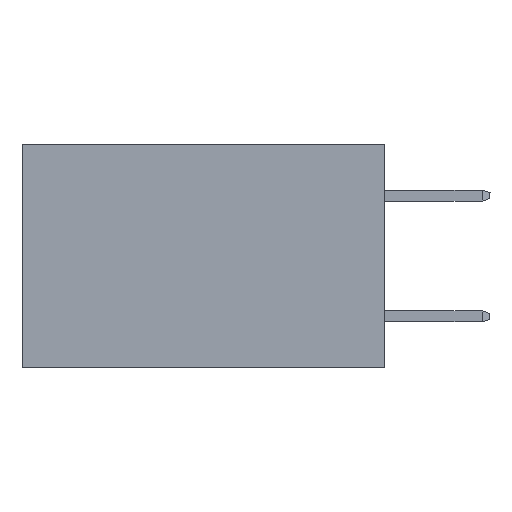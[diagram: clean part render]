
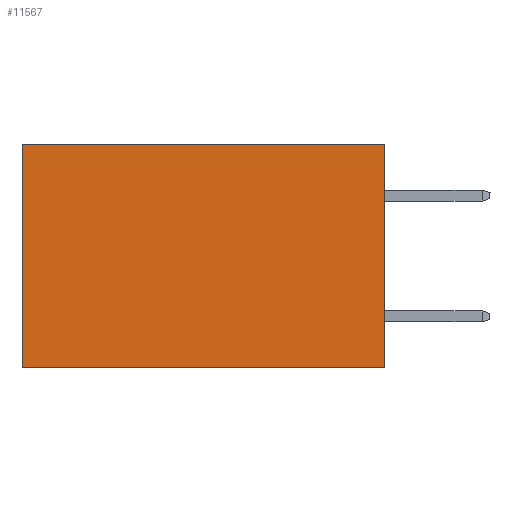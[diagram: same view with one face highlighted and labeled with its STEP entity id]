
A CAD part, left-side view. The second image highlights one B-rep face of the part: STEP entity #11567.
In plain terms, the highlighted planar face has unit normal (-1, 0, 0).
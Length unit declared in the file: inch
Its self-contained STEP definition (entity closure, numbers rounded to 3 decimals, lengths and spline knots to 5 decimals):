
#1437 = VERTEX_POINT ( 'NONE', #6724 ) ;
#1518 = VECTOR ( 'NONE', #14528, 39.37008 ) ;
#2049 = DIRECTION ( 'NONE',  ( 0., 0., -1. ) ) ;
#3207 = VECTOR ( 'NONE', #14059, 39.37008 ) ;
#3283 = VECTOR ( 'NONE', #7486, 39.37008 ) ;
#4358 = CARTESIAN_POINT ( 'NONE',  ( 0.298, 0.6, 0. ) ) ;
#4400 = EDGE_CURVE ( 'NONE', #15596, #13441, #5658, .T. ) ;
#4455 = AXIS2_PLACEMENT_3D ( 'NONE', #16062, #10477, #2049 ) ;
#5658 = LINE ( 'NONE', #14724, #1518 ) ;
#5954 = LINE ( 'NONE', #13129, #13966 ) ;
#5987 = VERTEX_POINT ( 'NONE', #13545 ) ;
#6137 = ORIENTED_EDGE ( 'NONE', *, *, #4400, .T. ) ;
#6401 = EDGE_CURVE ( 'NONE', #5987, #1437, #10658, .T. ) ;
#6724 = CARTESIAN_POINT ( 'NONE',  ( 0.298, 0., -0.37 ) ) ;
#7486 = DIRECTION ( 'NONE',  ( 0., 1., 0. ) ) ;
#7903 = EDGE_CURVE ( 'NONE', #5987, #15596, #5954, .T. ) ;
#8319 = ORIENTED_EDGE ( 'NONE', *, *, #14448, .F. ) ;
#9016 = PLANE ( 'NONE',  #4455 ) ;
#10477 = DIRECTION ( 'NONE',  ( 1., 0., 0. ) ) ;
#10658 = LINE ( 'NONE', #16275, #3207 ) ;
#10907 = ORIENTED_EDGE ( 'NONE', *, *, #6401, .F. ) ;
#11567 = ADVANCED_FACE ( 'NONE', ( #17803 ), #9016, .F. ) ;
#13129 = CARTESIAN_POINT ( 'NONE',  ( 0.298, 0., 0. ) ) ;
#13441 = VERTEX_POINT ( 'NONE', #15647 ) ;
#13545 = CARTESIAN_POINT ( 'NONE',  ( 0.298, 0., 0. ) ) ;
#13761 = DIRECTION ( 'NONE',  ( 0., 1., 0. ) ) ;
#13779 = ORIENTED_EDGE ( 'NONE', *, *, #7903, .T. ) ;
#13966 = VECTOR ( 'NONE', #13761, 39.37008 ) ;
#14059 = DIRECTION ( 'NONE',  ( 0., 0., -1. ) ) ;
#14448 = EDGE_CURVE ( 'NONE', #1437, #13441, #18161, .T. ) ;
#14528 = DIRECTION ( 'NONE',  ( 0., 0., -1. ) ) ;
#14613 = CARTESIAN_POINT ( 'NONE',  ( 0.298, 0., -0.37 ) ) ;
#14724 = CARTESIAN_POINT ( 'NONE',  ( 0.298, 0.6, 0. ) ) ;
#15091 = EDGE_LOOP ( 'NONE', ( #6137, #8319, #10907, #13779 ) ) ;
#15596 = VERTEX_POINT ( 'NONE', #4358 ) ;
#15647 = CARTESIAN_POINT ( 'NONE',  ( 0.298, 0.6, -0.37 ) ) ;
#16062 = CARTESIAN_POINT ( 'NONE',  ( 0.298, 0., 0. ) ) ;
#16275 = CARTESIAN_POINT ( 'NONE',  ( 0.298, 0., 0. ) ) ;
#17803 = FACE_OUTER_BOUND ( 'NONE', #15091, .T. ) ;
#18161 = LINE ( 'NONE', #14613, #3283 ) ;
